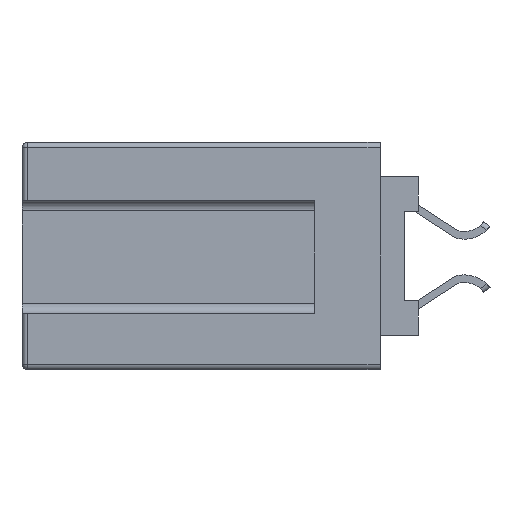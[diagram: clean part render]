
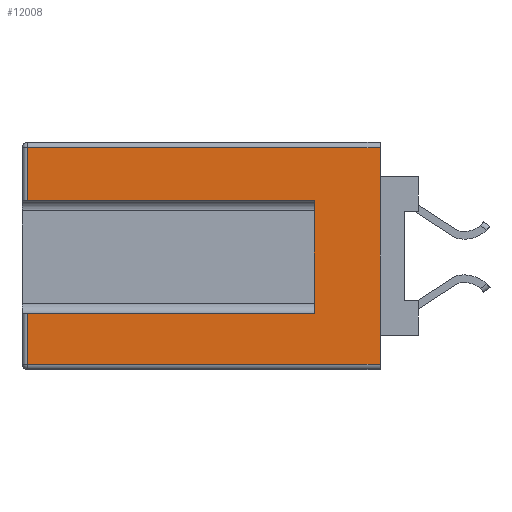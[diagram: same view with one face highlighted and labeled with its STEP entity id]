
A CAD part, left-side view. The second image highlights one B-rep face of the part: STEP entity #12008.
In plain terms, the highlighted planar face has unit normal (-1, 0, 0).
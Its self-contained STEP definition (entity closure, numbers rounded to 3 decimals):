
#273 = ORIENTED_EDGE ( 'NONE', *, *, #16663, .T. ) ;
#398 = LINE ( 'NONE', #35655, #33565 ) ;
#788 = CARTESIAN_POINT ( 'NONE',  ( 0., 15.3, 0. ) ) ;
#1308 = AXIS2_PLACEMENT_3D ( 'NONE', #14154, #39781, #11029 ) ;
#1351 = PLANE ( 'NONE',  #1308 ) ;
#2055 = VERTEX_POINT ( 'NONE', #40314 ) ;
#2457 = DIRECTION ( 'NONE',  ( 0., 0., -1. ) ) ;
#2716 = DIRECTION ( 'NONE',  ( 0., 1., 0. ) ) ;
#3753 = ORIENTED_EDGE ( 'NONE', *, *, #9417, .T. ) ;
#4267 = DIRECTION ( 'NONE',  ( 0., 1., 0. ) ) ;
#4651 = VECTOR ( 'NONE', #26857, 1000. ) ;
#6111 = EDGE_CURVE ( 'NONE', #2055, #33322, #16529, .T. ) ;
#7866 = DIRECTION ( 'NONE',  ( 0., -1., 0. ) ) ;
#8228 = EDGE_CURVE ( 'NONE', #33322, #8478, #18973, .T. ) ;
#8478 = VERTEX_POINT ( 'NONE', #39949 ) ;
#8660 = EDGE_CURVE ( 'NONE', #8478, #15811, #34010, .T. ) ;
#8910 = CARTESIAN_POINT ( 'NONE',  ( 0., 4.07, -2.28 ) ) ;
#9417 = EDGE_CURVE ( 'NONE', #15811, #20192, #29242, .T. ) ;
#9985 = VECTOR ( 'NONE', #21699, 1000. ) ;
#10363 = CARTESIAN_POINT ( 'NONE',  ( 0., 4.07, -6.68 ) ) ;
#10505 = VECTOR ( 'NONE', #2457, 1000. ) ;
#11029 = DIRECTION ( 'NONE',  ( 0., 0., -1. ) ) ;
#11596 = CARTESIAN_POINT ( 'NONE',  ( 0., 1.5, -8.68 ) ) ;
#12008 = ADVANCED_FACE ( 'NONE', ( #29896 ), #1351, .F. ) ;
#12440 = ORIENTED_EDGE ( 'NONE', *, *, #26977, .T. ) ;
#12456 = VERTEX_POINT ( 'NONE', #11596 ) ;
#13058 = VECTOR ( 'NONE', #22382, 1000. ) ;
#14153 = CARTESIAN_POINT ( 'NONE',  ( 0., 15.5, -8.68 ) ) ;
#14154 = CARTESIAN_POINT ( 'NONE',  ( 0., 15.5, 0. ) ) ;
#14572 = LINE ( 'NONE', #14153, #15967 ) ;
#14740 = ORIENTED_EDGE ( 'NONE', *, *, #8228, .T. ) ;
#15337 = EDGE_CURVE ( 'NONE', #27892, #12456, #31620, .T. ) ;
#15660 = VECTOR ( 'NONE', #38340, 1000. ) ;
#15811 = VERTEX_POINT ( 'NONE', #19530 ) ;
#15888 = CARTESIAN_POINT ( 'NONE',  ( 0., 15.3, 0. ) ) ;
#15964 = EDGE_LOOP ( 'NONE', ( #273, #27688, #17660, #12440, #22022, #14740, #16752, #3753 ) ) ;
#15967 = VECTOR ( 'NONE', #7866, 1000. ) ;
#16529 = LINE ( 'NONE', #788, #10505 ) ;
#16663 = EDGE_CURVE ( 'NONE', #20192, #40963, #31849, .T. ) ;
#16752 = ORIENTED_EDGE ( 'NONE', *, *, #8660, .T. ) ;
#17660 = ORIENTED_EDGE ( 'NONE', *, *, #15337, .F. ) ;
#18973 = LINE ( 'NONE', #8910, #9985 ) ;
#19530 = CARTESIAN_POINT ( 'NONE',  ( 0., 4.07, -6.68 ) ) ;
#19809 = CARTESIAN_POINT ( 'NONE',  ( 0., 15.3, -8.68 ) ) ;
#20192 = VERTEX_POINT ( 'NONE', #22653 ) ;
#21699 = DIRECTION ( 'NONE',  ( 0., -1., 0. ) ) ;
#22022 = ORIENTED_EDGE ( 'NONE', *, *, #6111, .T. ) ;
#22382 = DIRECTION ( 'NONE',  ( 0., 0., -1. ) ) ;
#22582 = EDGE_CURVE ( 'NONE', #40963, #12456, #14572, .T. ) ;
#22653 = CARTESIAN_POINT ( 'NONE',  ( 0., 15.3, -6.68 ) ) ;
#24802 = CARTESIAN_POINT ( 'NONE',  ( 0., 1.5, -0.2 ) ) ;
#25509 = CARTESIAN_POINT ( 'NONE',  ( 0., 1.5, 0. ) ) ;
#26857 = DIRECTION ( 'NONE',  ( 0., 0., -1. ) ) ;
#26977 = EDGE_CURVE ( 'NONE', #27892, #2055, #398, .T. ) ;
#27688 = ORIENTED_EDGE ( 'NONE', *, *, #22582, .T. ) ;
#27892 = VERTEX_POINT ( 'NONE', #24802 ) ;
#29242 = LINE ( 'NONE', #10363, #37186 ) ;
#29896 = FACE_OUTER_BOUND ( 'NONE', #15964, .T. ) ;
#31620 = LINE ( 'NONE', #25509, #15660 ) ;
#31849 = LINE ( 'NONE', #15888, #13058 ) ;
#33322 = VERTEX_POINT ( 'NONE', #35815 ) ;
#33565 = VECTOR ( 'NONE', #2716, 1000. ) ;
#33805 = CARTESIAN_POINT ( 'NONE',  ( 0., 4.07, -2.28 ) ) ;
#34010 = LINE ( 'NONE', #33805, #4651 ) ;
#35655 = CARTESIAN_POINT ( 'NONE',  ( 0., 15.5, -0.2 ) ) ;
#35815 = CARTESIAN_POINT ( 'NONE',  ( 0., 15.3, -2.28 ) ) ;
#37186 = VECTOR ( 'NONE', #4267, 1000. ) ;
#38340 = DIRECTION ( 'NONE',  ( 0., 0., -1. ) ) ;
#39781 = DIRECTION ( 'NONE',  ( 1., 0., 0. ) ) ;
#39949 = CARTESIAN_POINT ( 'NONE',  ( 0., 4.07, -2.28 ) ) ;
#40314 = CARTESIAN_POINT ( 'NONE',  ( 0., 15.3, -0.2 ) ) ;
#40963 = VERTEX_POINT ( 'NONE', #19809 ) ;
